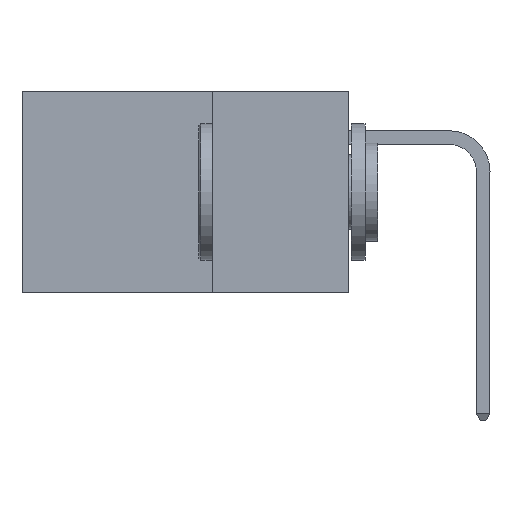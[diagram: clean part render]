
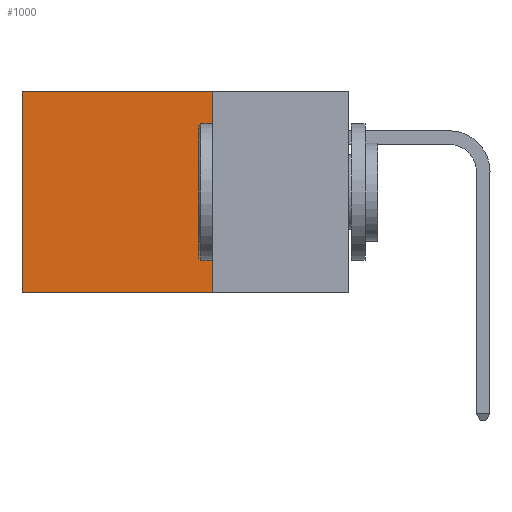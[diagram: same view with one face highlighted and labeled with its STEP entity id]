
A CAD part, left-side view. The second image highlights one B-rep face of the part: STEP entity #1000.
In plain terms, the highlighted planar face has unit normal (-1, 0, 0).
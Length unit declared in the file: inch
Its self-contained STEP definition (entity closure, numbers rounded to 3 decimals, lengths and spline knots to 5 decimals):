
#32 = CARTESIAN_POINT ( 'NONE',  ( 0.2875, 0.25, 0. ) ) ;
#311 = CARTESIAN_POINT ( 'NONE',  ( 0.2875, 0.25, 0. ) ) ;
#363 = FACE_OUTER_BOUND ( 'NONE', #3644, .T. ) ;
#526 = DIRECTION ( 'NONE',  ( 0., 1., 0. ) ) ;
#1000 = ADVANCED_FACE ( 'NONE', ( #363 ), #7594, .F. ) ;
#1448 = VECTOR ( 'NONE', #12428, 39.37008 ) ;
#1514 = VERTEX_POINT ( 'NONE', #10007 ) ;
#1703 = DIRECTION ( 'NONE',  ( 0., 1., 0. ) ) ;
#1929 = EDGE_CURVE ( 'NONE', #5517, #1514, #7543, .T. ) ;
#2055 = AXIS2_PLACEMENT_3D ( 'NONE', #32, #4911, #9703 ) ;
#2479 = ORIENTED_EDGE ( 'NONE', *, *, #1929, .T. ) ;
#3644 = EDGE_LOOP ( 'NONE', ( #4375, #13178, #3826, #2479 ) ) ;
#3826 = ORIENTED_EDGE ( 'NONE', *, *, #14095, .F. ) ;
#4007 = LINE ( 'NONE', #10527, #9542 ) ;
#4375 = ORIENTED_EDGE ( 'NONE', *, *, #6814, .T. ) ;
#4576 = VECTOR ( 'NONE', #1703, 39.37008 ) ;
#4726 = CARTESIAN_POINT ( 'NONE',  ( 0.2875, 0.25, 0. ) ) ;
#4729 = VERTEX_POINT ( 'NONE', #6324 ) ;
#4911 = DIRECTION ( 'NONE',  ( 1., 0., 0. ) ) ;
#4996 = EDGE_CURVE ( 'NONE', #4729, #8778, #10439, .T. ) ;
#5517 = VERTEX_POINT ( 'NONE', #10301 ) ;
#6324 = CARTESIAN_POINT ( 'NONE',  ( 0.2875, 0.25, -0.37 ) ) ;
#6814 = EDGE_CURVE ( 'NONE', #1514, #8778, #4007, .T. ) ;
#7218 = CARTESIAN_POINT ( 'NONE',  ( 0.2875, 0.6, -0.37 ) ) ;
#7543 = LINE ( 'NONE', #311, #4576 ) ;
#7594 = PLANE ( 'NONE',  #2055 ) ;
#7893 = VECTOR ( 'NONE', #526, 39.37008 ) ;
#8282 = DIRECTION ( 'NONE',  ( 0., 0., -1. ) ) ;
#8778 = VERTEX_POINT ( 'NONE', #7218 ) ;
#9542 = VECTOR ( 'NONE', #8282, 39.37008 ) ;
#9703 = DIRECTION ( 'NONE',  ( 0., 0., -1. ) ) ;
#10007 = CARTESIAN_POINT ( 'NONE',  ( 0.2875, 0.6, 0. ) ) ;
#10301 = CARTESIAN_POINT ( 'NONE',  ( 0.2875, 0.25, 0. ) ) ;
#10339 = LINE ( 'NONE', #4726, #1448 ) ;
#10439 = LINE ( 'NONE', #13876, #7893 ) ;
#10527 = CARTESIAN_POINT ( 'NONE',  ( 0.2875, 0.6, 0. ) ) ;
#12428 = DIRECTION ( 'NONE',  ( 0., 0., -1. ) ) ;
#13178 = ORIENTED_EDGE ( 'NONE', *, *, #4996, .F. ) ;
#13876 = CARTESIAN_POINT ( 'NONE',  ( 0.2875, 0.25, -0.37 ) ) ;
#14095 = EDGE_CURVE ( 'NONE', #5517, #4729, #10339, .T. ) ;
